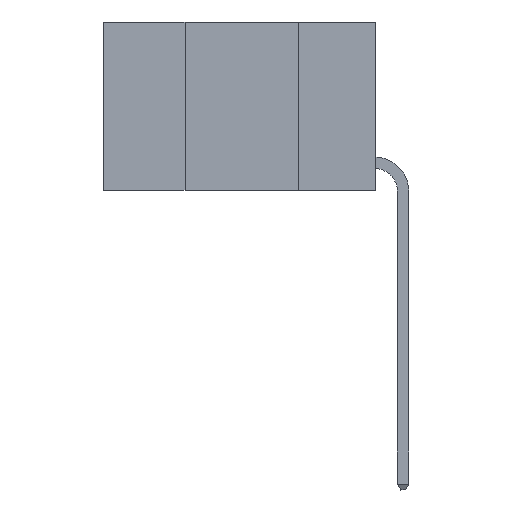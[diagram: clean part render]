
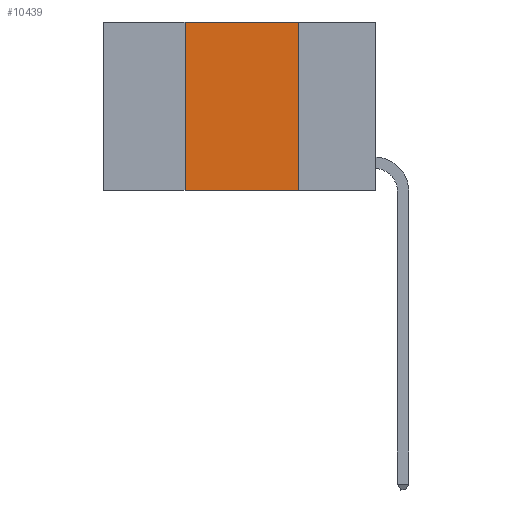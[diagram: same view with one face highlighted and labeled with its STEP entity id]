
A CAD part, left-side view. The second image highlights one B-rep face of the part: STEP entity #10439.
In plain terms, the highlighted planar face has unit normal (-1, 0, 0).
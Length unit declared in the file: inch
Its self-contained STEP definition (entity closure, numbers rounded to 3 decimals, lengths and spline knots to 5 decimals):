
#267 = CARTESIAN_POINT ( 'NONE',  ( 0., 0.42, -0.37 ) ) ;
#440 = LINE ( 'NONE', #11427, #5105 ) ;
#738 = DIRECTION ( 'NONE',  ( 0., -1., 0. ) ) ;
#991 = DIRECTION ( 'NONE',  ( 0., 0., -1. ) ) ;
#2624 = DIRECTION ( 'NONE',  ( 1., 0., 0. ) ) ;
#2700 = CARTESIAN_POINT ( 'NONE',  ( 0., 0.42, 0. ) ) ;
#3705 = PLANE ( 'NONE',  #11912 ) ;
#3819 = EDGE_CURVE ( 'NONE', #4302, #4353, #10980, .T. ) ;
#4302 = VERTEX_POINT ( 'NONE', #267 ) ;
#4353 = VERTEX_POINT ( 'NONE', #7503 ) ;
#4376 = EDGE_LOOP ( 'NONE', ( #5950, #7906, #9345, #9422 ) ) ;
#4414 = CARTESIAN_POINT ( 'NONE',  ( 0., 0.6, -0.37 ) ) ;
#4430 = VECTOR ( 'NONE', #738, 39.37008 ) ;
#4821 = EDGE_CURVE ( 'NONE', #11299, #8422, #440, .T. ) ;
#5105 = VECTOR ( 'NONE', #9483, 39.37008 ) ;
#5286 = LINE ( 'NONE', #8914, #4430 ) ;
#5950 = ORIENTED_EDGE ( 'NONE', *, *, #4821, .F. ) ;
#6150 = CARTESIAN_POINT ( 'NONE',  ( 0., 0.17, -0.37 ) ) ;
#7166 = EDGE_CURVE ( 'NONE', #4302, #8422, #10917, .T. ) ;
#7503 = CARTESIAN_POINT ( 'NONE',  ( 0., 0.42, 0. ) ) ;
#7558 = EDGE_CURVE ( 'NONE', #4353, #11299, #5286, .T. ) ;
#7906 = ORIENTED_EDGE ( 'NONE', *, *, #7558, .F. ) ;
#8182 = FACE_OUTER_BOUND ( 'NONE', #4376, .T. ) ;
#8206 = CARTESIAN_POINT ( 'NONE',  ( 0., 0.17, 0. ) ) ;
#8262 = VECTOR ( 'NONE', #11823, 39.37008 ) ;
#8422 = VERTEX_POINT ( 'NONE', #6150 ) ;
#8914 = CARTESIAN_POINT ( 'NONE',  ( 0., 0.6, 0. ) ) ;
#9345 = ORIENTED_EDGE ( 'NONE', *, *, #3819, .F. ) ;
#9422 = ORIENTED_EDGE ( 'NONE', *, *, #7166, .T. ) ;
#9483 = DIRECTION ( 'NONE',  ( 0., 0., -1. ) ) ;
#10269 = VECTOR ( 'NONE', #10311, 39.37008 ) ;
#10311 = DIRECTION ( 'NONE',  ( 0., 0., 1. ) ) ;
#10439 = ADVANCED_FACE ( 'NONE', ( #8182 ), #3705, .F. ) ;
#10917 = LINE ( 'NONE', #4414, #8262 ) ;
#10980 = LINE ( 'NONE', #2700, #10269 ) ;
#11299 = VERTEX_POINT ( 'NONE', #8206 ) ;
#11427 = CARTESIAN_POINT ( 'NONE',  ( 0., 0.17, 0. ) ) ;
#11810 = CARTESIAN_POINT ( 'NONE',  ( 0., 0.6, 0. ) ) ;
#11823 = DIRECTION ( 'NONE',  ( 0., -1., 0. ) ) ;
#11912 = AXIS2_PLACEMENT_3D ( 'NONE', #11810, #2624, #991 ) ;
